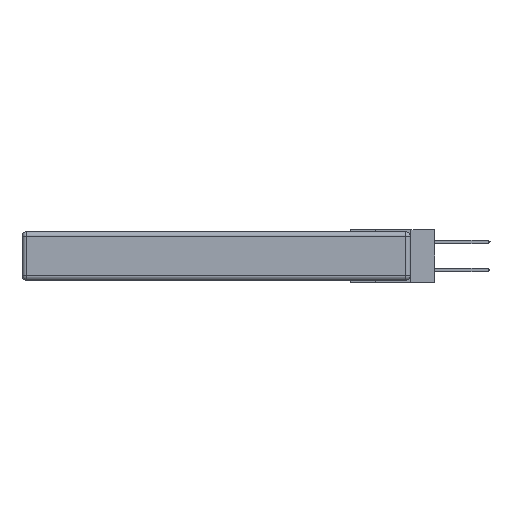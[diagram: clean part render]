
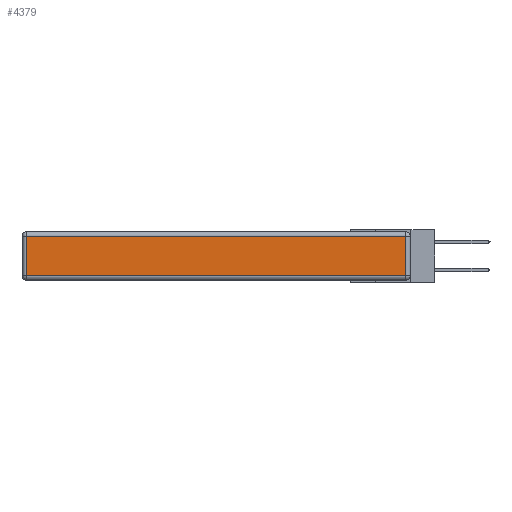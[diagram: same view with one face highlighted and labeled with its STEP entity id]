
A CAD part, left-side view. The second image highlights one B-rep face of the part: STEP entity #4379.
In plain terms, the highlighted planar face has unit normal (-1, 0, 0).
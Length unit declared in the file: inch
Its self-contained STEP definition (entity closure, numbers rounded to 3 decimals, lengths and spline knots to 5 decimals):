
#1269 = EDGE_CURVE ( 'NONE', #12034, #23088, #19687, .T. ) ;
#2707 = DIRECTION ( 'NONE',  ( 0., -1., 0. ) ) ;
#4335 = VECTOR ( 'NONE', #26721, 39.37008 ) ;
#4379 = ADVANCED_FACE ( 'NONE', ( #9370 ), #23395, .T. ) ;
#5018 = VERTEX_POINT ( 'NONE', #16249 ) ;
#6411 = ORIENTED_EDGE ( 'NONE', *, *, #9676, .T. ) ;
#9370 = FACE_OUTER_BOUND ( 'NONE', #9519, .T. ) ;
#9519 = EDGE_LOOP ( 'NONE', ( #19444, #12051, #30008, #6411 ) ) ;
#9676 = EDGE_CURVE ( 'NONE', #23088, #29871, #25134, .T. ) ;
#9852 = AXIS2_PLACEMENT_3D ( 'NONE', #11439, #14537, #19202 ) ;
#11439 = CARTESIAN_POINT ( 'NONE',  ( 0., 0., -0.343 ) ) ;
#11614 = CARTESIAN_POINT ( 'NONE',  ( 0., 0.03, -0.03 ) ) ;
#12034 = VERTEX_POINT ( 'NONE', #11614 ) ;
#12051 = ORIENTED_EDGE ( 'NONE', *, *, #26699, .T. ) ;
#13309 = CARTESIAN_POINT ( 'NONE',  ( 0., 2.72, -0.03 ) ) ;
#14537 = DIRECTION ( 'NONE',  ( -1., 0., 0. ) ) ;
#15087 = DIRECTION ( 'NONE',  ( 0., 0., -1. ) ) ;
#16134 = VECTOR ( 'NONE', #15087, 39.37008 ) ;
#16249 = CARTESIAN_POINT ( 'NONE',  ( 0., 0.03, -0.313 ) ) ;
#16904 = CARTESIAN_POINT ( 'NONE',  ( 0., 2.75, -0.03 ) ) ;
#18627 = CARTESIAN_POINT ( 'NONE',  ( 0., 0., -0.313 ) ) ;
#18883 = DIRECTION ( 'NONE',  ( 0., 0., 1. ) ) ;
#19202 = DIRECTION ( 'NONE',  ( 0., 0., 1. ) ) ;
#19314 = VECTOR ( 'NONE', #2707, 39.37008 ) ;
#19444 = ORIENTED_EDGE ( 'NONE', *, *, #20423, .T. ) ;
#19687 = LINE ( 'NONE', #16904, #4335 ) ;
#20177 = LINE ( 'NONE', #27947, #22793 ) ;
#20423 = EDGE_CURVE ( 'NONE', #29871, #5018, #26769, .T. ) ;
#22793 = VECTOR ( 'NONE', #18883, 39.37008 ) ;
#23088 = VERTEX_POINT ( 'NONE', #13309 ) ;
#23395 = PLANE ( 'NONE',  #9852 ) ;
#25134 = LINE ( 'NONE', #29393, #16134 ) ;
#25565 = CARTESIAN_POINT ( 'NONE',  ( 0., 2.72, -0.313 ) ) ;
#26699 = EDGE_CURVE ( 'NONE', #5018, #12034, #20177, .T. ) ;
#26721 = DIRECTION ( 'NONE',  ( 0., 1., 0. ) ) ;
#26769 = LINE ( 'NONE', #18627, #19314 ) ;
#27947 = CARTESIAN_POINT ( 'NONE',  ( 0., 0.03, -0.343 ) ) ;
#29393 = CARTESIAN_POINT ( 'NONE',  ( 0., 2.72, -0.343 ) ) ;
#29871 = VERTEX_POINT ( 'NONE', #25565 ) ;
#30008 = ORIENTED_EDGE ( 'NONE', *, *, #1269, .T. ) ;
